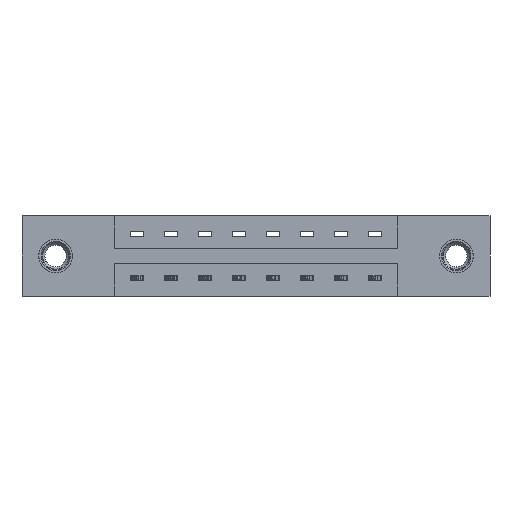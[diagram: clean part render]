
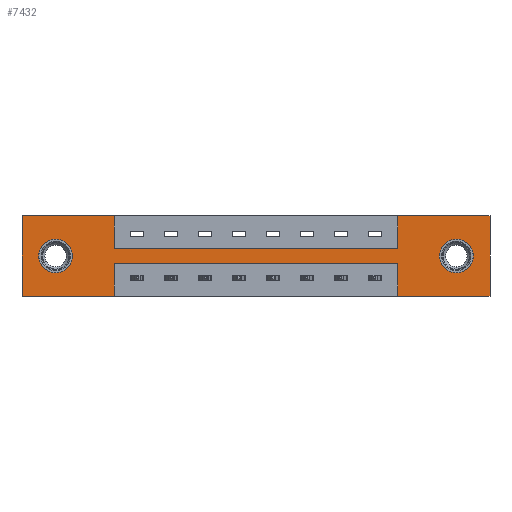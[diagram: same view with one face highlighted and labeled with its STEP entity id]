
A CAD part, front view. The second image highlights one B-rep face of the part: STEP entity #7432.
In plain terms, the highlighted planar face has unit normal (0, -1, 0).
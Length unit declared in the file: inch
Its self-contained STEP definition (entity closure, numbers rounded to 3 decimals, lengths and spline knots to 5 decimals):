
#189 = VERTEX_POINT ( 'NONE', #6331 ) ;
#227 = ORIENTED_EDGE ( 'NONE', *, *, #7228, .F. ) ;
#235 = EDGE_CURVE ( 'NONE', #6924, #6910, #3682, .T. ) ;
#688 = VECTOR ( 'NONE', #11129, 39.37008 ) ;
#924 = EDGE_CURVE ( 'NONE', #8872, #6924, #2826, .T. ) ;
#1142 = CARTESIAN_POINT ( 'NONE',  ( 0.155, 0., -0.185 ) ) ;
#1161 = LINE ( 'NONE', #10085, #9553 ) ;
#1219 = DIRECTION ( 'NONE',  ( 0., 0., -1. ) ) ;
#1484 = DIRECTION ( 'NONE',  ( 1., 0., 0. ) ) ;
#1488 = VECTOR ( 'NONE', #8271, 39.37008 ) ;
#1605 = VERTEX_POINT ( 'NONE', #9300 ) ;
#1791 = CARTESIAN_POINT ( 'NONE',  ( 2.154, 0., 0. ) ) ;
#1807 = VERTEX_POINT ( 'NONE', #8030 ) ;
#1808 = CARTESIAN_POINT ( 'NONE',  ( 0., 0., 0. ) ) ;
#1909 = ORIENTED_EDGE ( 'NONE', *, *, #5364, .F. ) ;
#1933 = CARTESIAN_POINT ( 'NONE',  ( 1.999, 0., -0.107 ) ) ;
#2051 = ORIENTED_EDGE ( 'NONE', *, *, #924, .F. ) ;
#2351 = DIRECTION ( 'NONE',  ( 0., 1., 0. ) ) ;
#2641 = FACE_OUTER_BOUND ( 'NONE', #2935, .T. ) ;
#2801 = CARTESIAN_POINT ( 'NONE',  ( 1.729, 0., -0.22 ) ) ;
#2826 = LINE ( 'NONE', #9391, #7652 ) ;
#2877 = VECTOR ( 'NONE', #10029, 39.37008 ) ;
#2913 = LINE ( 'NONE', #10903, #6023 ) ;
#2919 = CARTESIAN_POINT ( 'NONE',  ( 0.155, 0., -0.185 ) ) ;
#2935 = EDGE_LOOP ( 'NONE', ( #7393, #5483, #2051, #11002, #227, #5651, #4736, #3124, #1909, #6474, #5367, #5403 ) ) ;
#3008 = VERTEX_POINT ( 'NONE', #10834 ) ;
#3053 = EDGE_CURVE ( 'NONE', #1807, #7381, #2913, .T. ) ;
#3124 = ORIENTED_EDGE ( 'NONE', *, *, #11049, .F. ) ;
#3235 = CARTESIAN_POINT ( 'NONE',  ( 2.154, 0., 0. ) ) ;
#3240 = CARTESIAN_POINT ( 'NONE',  ( 0., 0., 0. ) ) ;
#3405 = LINE ( 'NONE', #3235, #5696 ) ;
#3409 = CARTESIAN_POINT ( 'NONE',  ( 2.154, 0., -0.37 ) ) ;
#3474 = VERTEX_POINT ( 'NONE', #1791 ) ;
#3682 = LINE ( 'NONE', #5405, #6382 ) ;
#3835 = EDGE_CURVE ( 'NONE', #6910, #1807, #5730, .T. ) ;
#3860 = AXIS2_PLACEMENT_3D ( 'NONE', #8434, #10348, #4921 ) ;
#3872 = DIRECTION ( 'NONE',  ( 1., 0., 0. ) ) ;
#3879 = EDGE_CURVE ( 'NONE', #3008, #189, #5582, .T. ) ;
#3920 = VERTEX_POINT ( 'NONE', #8805 ) ;
#3954 = LINE ( 'NONE', #4729, #7787 ) ;
#4034 = AXIS2_PLACEMENT_3D ( 'NONE', #2919, #11242, #5882 ) ;
#4111 = VERTEX_POINT ( 'NONE', #5752 ) ;
#4221 = VECTOR ( 'NONE', #3872, 39.37008 ) ;
#4377 = LINE ( 'NONE', #1808, #9142 ) ;
#4451 = EDGE_CURVE ( 'NONE', #5294, #7606, #10585, .T. ) ;
#4618 = CARTESIAN_POINT ( 'NONE',  ( 1.729, 0., 0. ) ) ;
#4665 = VERTEX_POINT ( 'NONE', #1933 ) ;
#4729 = CARTESIAN_POINT ( 'NONE',  ( 0., 0., -0.37 ) ) ;
#4736 = ORIENTED_EDGE ( 'NONE', *, *, #4451, .F. ) ;
#4866 = DIRECTION ( 'NONE',  ( 0., -1., 0. ) ) ;
#4873 = VECTOR ( 'NONE', #1484, 39.37008 ) ;
#4921 = DIRECTION ( 'NONE',  ( 0., 0., -1. ) ) ;
#5087 = LINE ( 'NONE', #9249, #4221 ) ;
#5237 = VERTEX_POINT ( 'NONE', #6555 ) ;
#5294 = VERTEX_POINT ( 'NONE', #5571 ) ;
#5341 = CARTESIAN_POINT ( 'NONE',  ( 0.425, 0., -0.22 ) ) ;
#5364 = EDGE_CURVE ( 'NONE', #189, #3920, #7169, .T. ) ;
#5367 = ORIENTED_EDGE ( 'NONE', *, *, #9717, .F. ) ;
#5403 = ORIENTED_EDGE ( 'NONE', *, *, #3053, .F. ) ;
#5405 = CARTESIAN_POINT ( 'NONE',  ( 0.425, 0., -0.22 ) ) ;
#5483 = ORIENTED_EDGE ( 'NONE', *, *, #235, .F. ) ;
#5571 = CARTESIAN_POINT ( 'NONE',  ( 1.729, 0., -0.15 ) ) ;
#5582 = LINE ( 'NONE', #3240, #4873 ) ;
#5651 = ORIENTED_EDGE ( 'NONE', *, *, #10115, .F. ) ;
#5696 = VECTOR ( 'NONE', #10367, 39.37008 ) ;
#5703 = CARTESIAN_POINT ( 'NONE',  ( 0., 0., -0.37 ) ) ;
#5730 = LINE ( 'NONE', #6430, #1488 ) ;
#5752 = CARTESIAN_POINT ( 'NONE',  ( 0.155, 0., -0.107 ) ) ;
#5882 = DIRECTION ( 'NONE',  ( 0., 0., 1. ) ) ;
#5946 = EDGE_CURVE ( 'NONE', #4665, #1605, #8788, .T. ) ;
#6023 = VECTOR ( 'NONE', #8219, 39.37008 ) ;
#6331 = CARTESIAN_POINT ( 'NONE',  ( 0.425, 0., 0. ) ) ;
#6382 = VECTOR ( 'NONE', #10653, 39.37008 ) ;
#6430 = CARTESIAN_POINT ( 'NONE',  ( 0.425, 0., -0.37 ) ) ;
#6474 = ORIENTED_EDGE ( 'NONE', *, *, #3879, .F. ) ;
#6555 = CARTESIAN_POINT ( 'NONE',  ( 0.155, 0., -0.263 ) ) ;
#6569 = EDGE_CURVE ( 'NONE', #5237, #4111, #7562, .T. ) ;
#6597 = DIRECTION ( 'NONE',  ( -1., 0., 0. ) ) ;
#6910 = VERTEX_POINT ( 'NONE', #5341 ) ;
#6924 = VERTEX_POINT ( 'NONE', #2801 ) ;
#7169 = LINE ( 'NONE', #8564, #688 ) ;
#7228 = EDGE_CURVE ( 'NONE', #3474, #8513, #3405, .T. ) ;
#7381 = VERTEX_POINT ( 'NONE', #10190 ) ;
#7393 = ORIENTED_EDGE ( 'NONE', *, *, #3835, .F. ) ;
#7431 = DIRECTION ( 'NONE',  ( 0., 1., 0. ) ) ;
#7432 = ADVANCED_FACE ( 'NONE', ( #11178, #9685, #2641 ), #7529, .T. ) ;
#7529 = PLANE ( 'NONE',  #9524 ) ;
#7562 = CIRCLE ( 'NONE', #8480, 0.078 ) ;
#7606 = VERTEX_POINT ( 'NONE', #10829 ) ;
#7652 = VECTOR ( 'NONE', #7668, 39.37008 ) ;
#7668 = DIRECTION ( 'NONE',  ( 0., 0., 1. ) ) ;
#7787 = VECTOR ( 'NONE', #6597, 39.37008 ) ;
#7798 = CARTESIAN_POINT ( 'NONE',  ( 1.999, 0., -0.185 ) ) ;
#8030 = CARTESIAN_POINT ( 'NONE',  ( 0.425, 0., -0.37 ) ) ;
#8140 = ORIENTED_EDGE ( 'NONE', *, *, #5946, .T. ) ;
#8219 = DIRECTION ( 'NONE',  ( -1., 0., 0. ) ) ;
#8238 = DIRECTION ( 'NONE',  ( 0., 0., 1. ) ) ;
#8271 = DIRECTION ( 'NONE',  ( 0., 0., -1. ) ) ;
#8273 = DIRECTION ( 'NONE',  ( 1., 0., 0. ) ) ;
#8320 = CIRCLE ( 'NONE', #11156, 0.078 ) ;
#8434 = CARTESIAN_POINT ( 'NONE',  ( 1.999, 0., -0.185 ) ) ;
#8457 = CIRCLE ( 'NONE', #4034, 0.078 ) ;
#8480 = AXIS2_PLACEMENT_3D ( 'NONE', #1142, #7431, #9192 ) ;
#8496 = EDGE_LOOP ( 'NONE', ( #11487, #10959 ) ) ;
#8513 = VERTEX_POINT ( 'NONE', #3409 ) ;
#8564 = CARTESIAN_POINT ( 'NONE',  ( 0.425, 0., 0. ) ) ;
#8766 = CARTESIAN_POINT ( 'NONE',  ( 1.729, 0., -0.37 ) ) ;
#8788 = CIRCLE ( 'NONE', #3860, 0.078 ) ;
#8805 = CARTESIAN_POINT ( 'NONE',  ( 0.425, 0., -0.15 ) ) ;
#8872 = VERTEX_POINT ( 'NONE', #8766 ) ;
#9142 = VECTOR ( 'NONE', #8238, 39.37008 ) ;
#9192 = DIRECTION ( 'NONE',  ( 0., 0., 1. ) ) ;
#9226 = ORIENTED_EDGE ( 'NONE', *, *, #10315, .T. ) ;
#9249 = CARTESIAN_POINT ( 'NONE',  ( 0.425, 0., -0.15 ) ) ;
#9286 = EDGE_CURVE ( 'NONE', #4111, #5237, #8457, .T. ) ;
#9300 = CARTESIAN_POINT ( 'NONE',  ( 1.999, 0., -0.263 ) ) ;
#9391 = CARTESIAN_POINT ( 'NONE',  ( 1.729, 0., -0.37 ) ) ;
#9524 = AXIS2_PLACEMENT_3D ( 'NONE', #5703, #4866, #1219 ) ;
#9553 = VECTOR ( 'NONE', #8273, 39.37008 ) ;
#9561 = DIRECTION ( 'NONE',  ( 0., 0., -1. ) ) ;
#9685 = FACE_BOUND ( 'NONE', #8496, .T. ) ;
#9717 = EDGE_CURVE ( 'NONE', #7381, #3008, #4377, .T. ) ;
#10029 = DIRECTION ( 'NONE',  ( 0., 0., 1. ) ) ;
#10085 = CARTESIAN_POINT ( 'NONE',  ( 0., 0., 0. ) ) ;
#10115 = EDGE_CURVE ( 'NONE', #7606, #3474, #1161, .T. ) ;
#10190 = CARTESIAN_POINT ( 'NONE',  ( 0., 0., -0.37 ) ) ;
#10281 = EDGE_LOOP ( 'NONE', ( #8140, #9226 ) ) ;
#10315 = EDGE_CURVE ( 'NONE', #1605, #4665, #8320, .T. ) ;
#10348 = DIRECTION ( 'NONE',  ( 0., 1., 0. ) ) ;
#10367 = DIRECTION ( 'NONE',  ( 0., 0., -1. ) ) ;
#10585 = LINE ( 'NONE', #4618, #2877 ) ;
#10653 = DIRECTION ( 'NONE',  ( -1., 0., 0. ) ) ;
#10829 = CARTESIAN_POINT ( 'NONE',  ( 1.729, 0., 0. ) ) ;
#10834 = CARTESIAN_POINT ( 'NONE',  ( 0., 0., 0. ) ) ;
#10903 = CARTESIAN_POINT ( 'NONE',  ( 0., 0., -0.37 ) ) ;
#10959 = ORIENTED_EDGE ( 'NONE', *, *, #6569, .T. ) ;
#11002 = ORIENTED_EDGE ( 'NONE', *, *, #11267, .F. ) ;
#11049 = EDGE_CURVE ( 'NONE', #3920, #5294, #5087, .T. ) ;
#11129 = DIRECTION ( 'NONE',  ( 0., 0., -1. ) ) ;
#11156 = AXIS2_PLACEMENT_3D ( 'NONE', #7798, #2351, #9561 ) ;
#11178 = FACE_BOUND ( 'NONE', #10281, .T. ) ;
#11242 = DIRECTION ( 'NONE',  ( 0., 1., 0. ) ) ;
#11267 = EDGE_CURVE ( 'NONE', #8513, #8872, #3954, .T. ) ;
#11487 = ORIENTED_EDGE ( 'NONE', *, *, #9286, .T. ) ;
